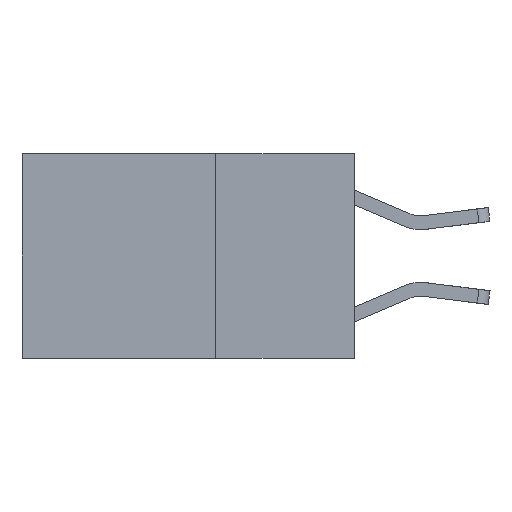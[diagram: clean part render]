
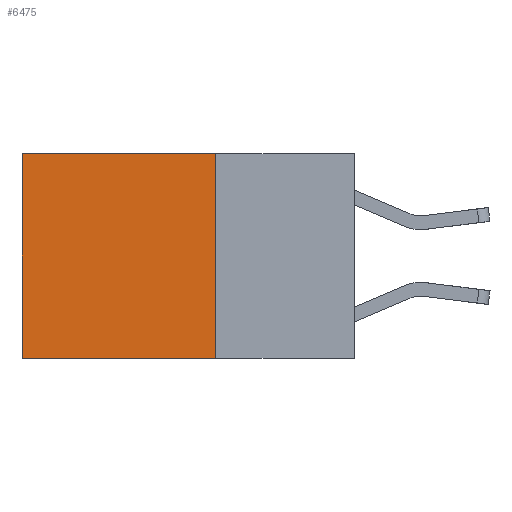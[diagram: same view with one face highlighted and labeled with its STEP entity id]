
A CAD part, left-side view. The second image highlights one B-rep face of the part: STEP entity #6475.
In plain terms, the highlighted planar face has unit normal (-1, 0, 0).
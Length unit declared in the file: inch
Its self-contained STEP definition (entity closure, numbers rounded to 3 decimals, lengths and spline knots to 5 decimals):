
#380 = LINE ( 'NONE', #9557, #9573 ) ;
#492 = VERTEX_POINT ( 'NONE', #8411 ) ;
#626 = VERTEX_POINT ( 'NONE', #8166 ) ;
#734 = AXIS2_PLACEMENT_3D ( 'NONE', #8354, #6003, #1612 ) ;
#1086 = LINE ( 'NONE', #9485, #8829 ) ;
#1612 = DIRECTION ( 'NONE',  ( 0., 0., -1. ) ) ;
#1738 = ORIENTED_EDGE ( 'NONE', *, *, #3261, .F. ) ;
#2250 = DIRECTION ( 'NONE',  ( 0., 1., 0. ) ) ;
#2795 = VERTEX_POINT ( 'NONE', #7923 ) ;
#3261 = EDGE_CURVE ( 'NONE', #492, #2795, #380, .T. ) ;
#3393 = VECTOR ( 'NONE', #4677, 39.37008 ) ;
#3950 = CARTESIAN_POINT ( 'NONE',  ( 0.2625, 0.6, 0. ) ) ;
#4260 = LINE ( 'NONE', #7506, #9167 ) ;
#4574 = VERTEX_POINT ( 'NONE', #8973 ) ;
#4610 = FACE_OUTER_BOUND ( 'NONE', #6697, .T. ) ;
#4677 = DIRECTION ( 'NONE',  ( 0., 0., -1. ) ) ;
#4846 = EDGE_CURVE ( 'NONE', #626, #4574, #5309, .T. ) ;
#5208 = PLANE ( 'NONE',  #734 ) ;
#5309 = LINE ( 'NONE', #3950, #3393 ) ;
#5353 = ORIENTED_EDGE ( 'NONE', *, *, #4846, .T. ) ;
#6003 = DIRECTION ( 'NONE',  ( 1., 0., 0. ) ) ;
#6474 = DIRECTION ( 'NONE',  ( 0., 1., 0. ) ) ;
#6475 = ADVANCED_FACE ( 'NONE', ( #4610 ), #5208, .F. ) ;
#6697 = EDGE_LOOP ( 'NONE', ( #5353, #9487, #1738, #7760 ) ) ;
#6881 = EDGE_CURVE ( 'NONE', #492, #626, #4260, .T. ) ;
#7506 = CARTESIAN_POINT ( 'NONE',  ( 0.2625, 0.25, 0. ) ) ;
#7760 = ORIENTED_EDGE ( 'NONE', *, *, #6881, .T. ) ;
#7923 = CARTESIAN_POINT ( 'NONE',  ( 0.2625, 0.25, -0.37 ) ) ;
#8166 = CARTESIAN_POINT ( 'NONE',  ( 0.2625, 0.6, 0. ) ) ;
#8354 = CARTESIAN_POINT ( 'NONE',  ( 0.2625, 0.25, 0. ) ) ;
#8371 = EDGE_CURVE ( 'NONE', #2795, #4574, #1086, .T. ) ;
#8411 = CARTESIAN_POINT ( 'NONE',  ( 0.2625, 0.25, 0. ) ) ;
#8829 = VECTOR ( 'NONE', #6474, 39.37008 ) ;
#8973 = CARTESIAN_POINT ( 'NONE',  ( 0.2625, 0.6, -0.37 ) ) ;
#9167 = VECTOR ( 'NONE', #2250, 39.37008 ) ;
#9408 = DIRECTION ( 'NONE',  ( 0., 0., -1. ) ) ;
#9485 = CARTESIAN_POINT ( 'NONE',  ( 0.2625, 0.25, -0.37 ) ) ;
#9487 = ORIENTED_EDGE ( 'NONE', *, *, #8371, .F. ) ;
#9557 = CARTESIAN_POINT ( 'NONE',  ( 0.2625, 0.25, 0. ) ) ;
#9573 = VECTOR ( 'NONE', #9408, 39.37008 ) ;
